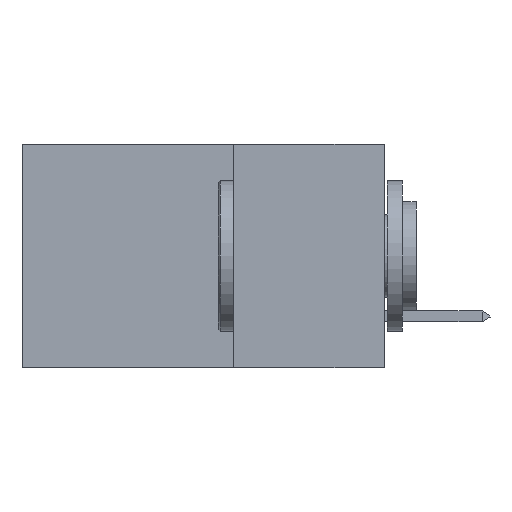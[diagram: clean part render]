
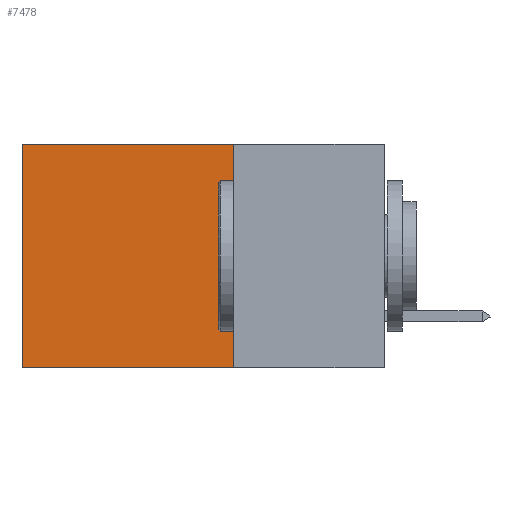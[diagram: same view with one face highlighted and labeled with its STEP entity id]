
A CAD part, left-side view. The second image highlights one B-rep face of the part: STEP entity #7478.
In plain terms, the highlighted planar face has unit normal (-1, 0, 0).
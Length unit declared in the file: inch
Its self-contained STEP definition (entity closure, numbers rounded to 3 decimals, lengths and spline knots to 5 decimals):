
#453 = ORIENTED_EDGE ( 'NONE', *, *, #17496, .T. ) ;
#1233 = CARTESIAN_POINT ( 'NONE',  ( 0.2875, 0.25, -0.37 ) ) ;
#1529 = VERTEX_POINT ( 'NONE', #8580 ) ;
#1885 = EDGE_CURVE ( 'NONE', #1529, #9056, #4125, .T. ) ;
#2594 = LINE ( 'NONE', #12403, #10577 ) ;
#3790 = DIRECTION ( 'NONE',  ( 1., 0., 0. ) ) ;
#4069 = DIRECTION ( 'NONE',  ( 0., 1., 0. ) ) ;
#4125 = LINE ( 'NONE', #10917, #16500 ) ;
#5216 = ORIENTED_EDGE ( 'NONE', *, *, #11957, .T. ) ;
#6631 = DIRECTION ( 'NONE',  ( 0., 1., 0. ) ) ;
#6980 = CARTESIAN_POINT ( 'NONE',  ( 0.2875, 0.25, 0. ) ) ;
#7478 = ADVANCED_FACE ( 'NONE', ( #10296 ), #17199, .F. ) ;
#7734 = LINE ( 'NONE', #10022, #11458 ) ;
#8507 = CARTESIAN_POINT ( 'NONE',  ( 0.2875, 0.6, -0.37 ) ) ;
#8580 = CARTESIAN_POINT ( 'NONE',  ( 0.2875, 0.25, 0. ) ) ;
#8582 = VERTEX_POINT ( 'NONE', #16481 ) ;
#8752 = VERTEX_POINT ( 'NONE', #8507 ) ;
#9056 = VERTEX_POINT ( 'NONE', #1233 ) ;
#9981 = EDGE_LOOP ( 'NONE', ( #5216, #16007, #13730, #453 ) ) ;
#10022 = CARTESIAN_POINT ( 'NONE',  ( 0.2875, 0.6, 0. ) ) ;
#10296 = FACE_OUTER_BOUND ( 'NONE', #9981, .T. ) ;
#10577 = VECTOR ( 'NONE', #6631, 39.37008 ) ;
#10917 = CARTESIAN_POINT ( 'NONE',  ( 0.2875, 0.25, 0. ) ) ;
#11369 = DIRECTION ( 'NONE',  ( 0., 0., -1. ) ) ;
#11458 = VECTOR ( 'NONE', #11589, 39.37008 ) ;
#11589 = DIRECTION ( 'NONE',  ( 0., 0., -1. ) ) ;
#11957 = EDGE_CURVE ( 'NONE', #8582, #8752, #7734, .T. ) ;
#12403 = CARTESIAN_POINT ( 'NONE',  ( 0.2875, 0.25, 0. ) ) ;
#13730 = ORIENTED_EDGE ( 'NONE', *, *, #1885, .F. ) ;
#14141 = EDGE_CURVE ( 'NONE', #9056, #8752, #18199, .T. ) ;
#15376 = DIRECTION ( 'NONE',  ( 0., 0., -1. ) ) ;
#15396 = VECTOR ( 'NONE', #4069, 39.37008 ) ;
#16007 = ORIENTED_EDGE ( 'NONE', *, *, #14141, .F. ) ;
#16481 = CARTESIAN_POINT ( 'NONE',  ( 0.2875, 0.6, 0. ) ) ;
#16500 = VECTOR ( 'NONE', #15376, 39.37008 ) ;
#17199 = PLANE ( 'NONE',  #18817 ) ;
#17496 = EDGE_CURVE ( 'NONE', #1529, #8582, #2594, .T. ) ;
#17519 = CARTESIAN_POINT ( 'NONE',  ( 0.2875, 0.25, -0.37 ) ) ;
#18199 = LINE ( 'NONE', #17519, #15396 ) ;
#18817 = AXIS2_PLACEMENT_3D ( 'NONE', #6980, #3790, #11369 ) ;
